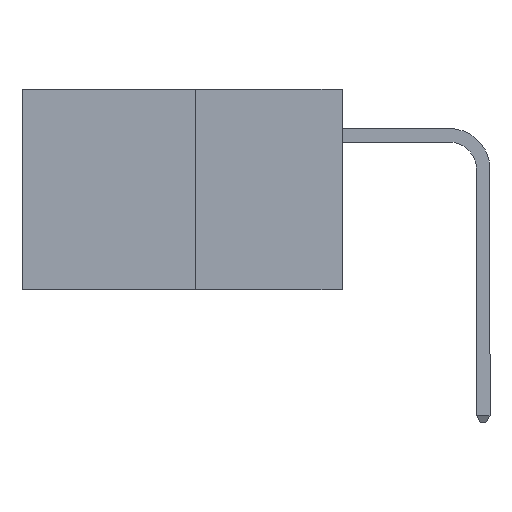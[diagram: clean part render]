
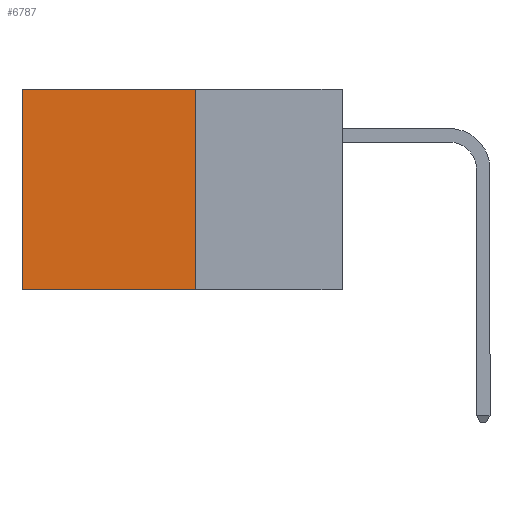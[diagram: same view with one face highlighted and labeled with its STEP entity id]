
A CAD part, left-side view. The second image highlights one B-rep face of the part: STEP entity #6787.
In plain terms, the highlighted planar face has unit normal (-1, 0, 0).
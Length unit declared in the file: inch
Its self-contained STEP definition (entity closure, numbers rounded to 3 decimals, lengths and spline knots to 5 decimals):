
#240 = LINE ( 'NONE', #13477, #19331 ) ;
#500 = DIRECTION ( 'NONE',  ( 0., 0., -1. ) ) ;
#1286 = DIRECTION ( 'NONE',  ( 0., 0., -1. ) ) ;
#1453 = LINE ( 'NONE', #9089, #5887 ) ;
#1553 = EDGE_CURVE ( 'NONE', #4854, #7001, #1453, .T. ) ;
#2905 = ORIENTED_EDGE ( 'NONE', *, *, #7503, .F. ) ;
#2995 = ORIENTED_EDGE ( 'NONE', *, *, #1553, .F. ) ;
#3413 = VECTOR ( 'NONE', #17850, 39.37008 ) ;
#4559 = LINE ( 'NONE', #17701, #3413 ) ;
#4854 = VERTEX_POINT ( 'NONE', #12412 ) ;
#5187 = EDGE_CURVE ( 'NONE', #5563, #15427, #240, .T. ) ;
#5563 = VERTEX_POINT ( 'NONE', #19643 ) ;
#5887 = VECTOR ( 'NONE', #9156, 39.37008 ) ;
#6787 = ADVANCED_FACE ( 'NONE', ( #7215 ), #21454, .F. ) ;
#7001 = VERTEX_POINT ( 'NONE', #13011 ) ;
#7215 = FACE_OUTER_BOUND ( 'NONE', #9537, .T. ) ;
#7503 = EDGE_CURVE ( 'NONE', #7001, #15427, #4559, .T. ) ;
#7620 = CARTESIAN_POINT ( 'NONE',  ( 0.277, 0.27, 0. ) ) ;
#8042 = ORIENTED_EDGE ( 'NONE', *, *, #21047, .T. ) ;
#9089 = CARTESIAN_POINT ( 'NONE',  ( 0.277, 0.27, -0.37 ) ) ;
#9156 = DIRECTION ( 'NONE',  ( 0., 0., -1. ) ) ;
#9537 = EDGE_LOOP ( 'NONE', ( #20776, #2905, #2995, #8042 ) ) ;
#10376 = VECTOR ( 'NONE', #14945, 39.37008 ) ;
#12412 = CARTESIAN_POINT ( 'NONE',  ( 0.277, 0.27, 0. ) ) ;
#12430 = DIRECTION ( 'NONE',  ( 1., 0., 0. ) ) ;
#13011 = CARTESIAN_POINT ( 'NONE',  ( 0.277, 0.27, -0.37 ) ) ;
#13477 = CARTESIAN_POINT ( 'NONE',  ( 0.277, 0.59, -0.37 ) ) ;
#14741 = LINE ( 'NONE', #7620, #10376 ) ;
#14945 = DIRECTION ( 'NONE',  ( 0., 1., 0. ) ) ;
#15427 = VERTEX_POINT ( 'NONE', #19625 ) ;
#17701 = CARTESIAN_POINT ( 'NONE',  ( 0.277, 0.27, -0.37 ) ) ;
#17850 = DIRECTION ( 'NONE',  ( 0., 1., 0. ) ) ;
#19331 = VECTOR ( 'NONE', #500, 39.37008 ) ;
#19625 = CARTESIAN_POINT ( 'NONE',  ( 0.277, 0.59, -0.37 ) ) ;
#19643 = CARTESIAN_POINT ( 'NONE',  ( 0.277, 0.59, 0. ) ) ;
#20776 = ORIENTED_EDGE ( 'NONE', *, *, #5187, .T. ) ;
#21047 = EDGE_CURVE ( 'NONE', #4854, #5563, #14741, .T. ) ;
#21454 = PLANE ( 'NONE',  #22959 ) ;
#22959 = AXIS2_PLACEMENT_3D ( 'NONE', #23368, #12430, #1286 ) ;
#23368 = CARTESIAN_POINT ( 'NONE',  ( 0.277, 0.27, -0.37 ) ) ;
